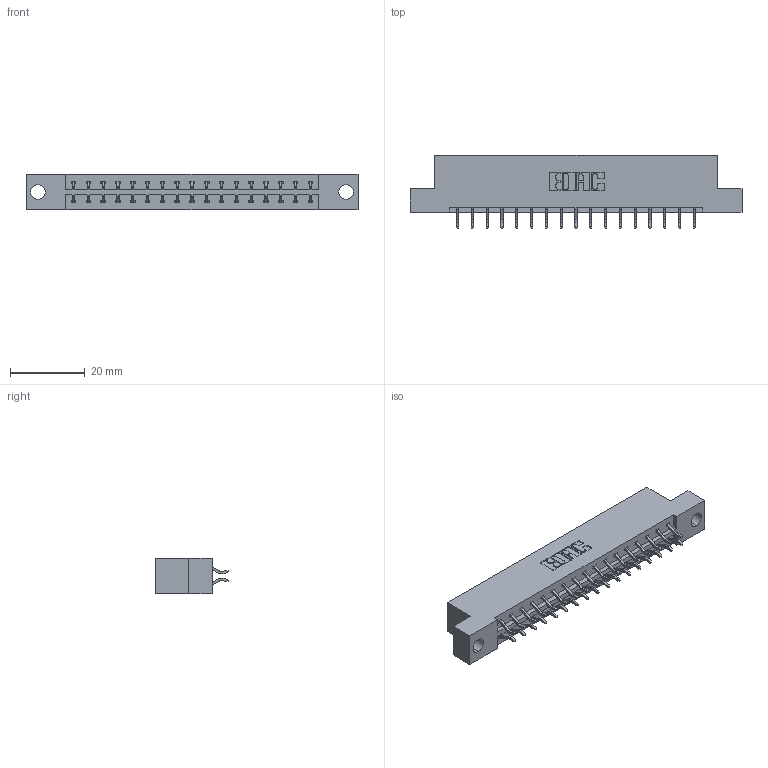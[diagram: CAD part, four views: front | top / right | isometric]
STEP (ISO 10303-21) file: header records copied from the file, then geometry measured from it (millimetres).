
FILE_DESCRIPTION (( 'STEP AP203' ), '1' );
FILE_NAME ('833-034-556-204.STEP', '2020-06-02T23:13:45', ( '' ), ( '' ), 'SwSTEP 2.0', 'SolidWorks 2020', '' );
FILE_SCHEMA (( 'CONFIG_CONTROL_DESIGN' ));
Length unit declared in the file: inch
Products named in the file (3): 833 Part_Flush - .156 Dia - TH; 345-292-001_556 Tail; 833-034-556-204
Assembly tree (35 placements, depth 2):
  833-034-556-204
    833 Part_Flush - .156 Dia - TH
    345-292-001_556 Tail  x34
Bounding box: 88.9 x 19.57 x 9.4 mm (x, y, z)
Volume: 8753.2 mm3; surface area: 9845.7 mm2
Topology: 35 solids, 35 shells, 2086 faces, 6193 edges, 4082 vertices
Faces by surface type: plane 1430, cylinder 656
Entity records: 14393 total; most frequent: CARTESIAN_POINT 2430, ORIENTED_EDGE 2354, DIRECTION 2109, EDGE_CURVE 1177, VECTOR 1041, LINE 1041, VERTEX_POINT 782, AXIS2_PLACEMENT_3D 534
